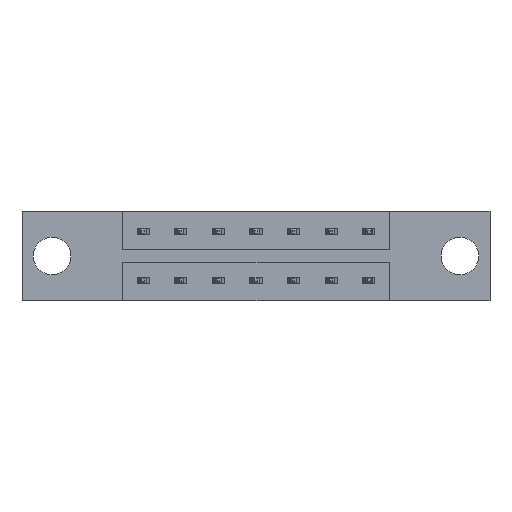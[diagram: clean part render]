
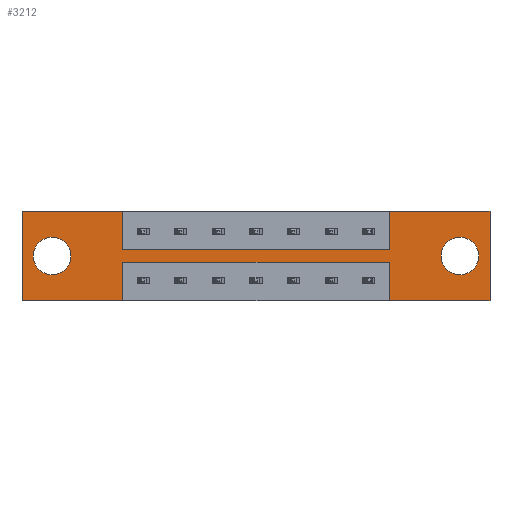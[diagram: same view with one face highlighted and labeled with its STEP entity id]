
A CAD part, front view. The second image highlights one B-rep face of the part: STEP entity #3212.
In plain terms, the highlighted planar face has unit normal (0, -1, 0).
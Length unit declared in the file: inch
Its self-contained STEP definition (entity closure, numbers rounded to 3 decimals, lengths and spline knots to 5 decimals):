
#24 = AXIS2_PLACEMENT_3D ( 'NONE', #7411, #3484, #8070 ) ;
#127 = VECTOR ( 'NONE', #6315, 39.37008 ) ;
#329 = CARTESIAN_POINT ( 'NONE',  ( 1.94, 0., 0. ) ) ;
#399 = VECTOR ( 'NONE', #4241, 39.37008 ) ;
#413 = VERTEX_POINT ( 'NONE', #4636 ) ;
#433 = DIRECTION ( 'NONE',  ( 0., 0., -1. ) ) ;
#529 = CARTESIAN_POINT ( 'NONE',  ( 1.5225, 0., -0.1585 ) ) ;
#573 = VECTOR ( 'NONE', #3287, 39.37008 ) ;
#631 = CIRCLE ( 'NONE', #5650, 0.078 ) ;
#705 = CARTESIAN_POINT ( 'NONE',  ( 1.815, 0., -0.107 ) ) ;
#706 = VERTEX_POINT ( 'NONE', #7564 ) ;
#843 = CARTESIAN_POINT ( 'NONE',  ( 0., 0., -0.37 ) ) ;
#888 = EDGE_LOOP ( 'NONE', ( #7225, #8269 ) ) ;
#948 = LINE ( 'NONE', #6165, #7922 ) ;
#1078 = DIRECTION ( 'NONE',  ( 0., 0., -1. ) ) ;
#1175 = DIRECTION ( 'NONE',  ( -1., 0., 0. ) ) ;
#1216 = DIRECTION ( 'NONE',  ( 0., 1., 0. ) ) ;
#1270 = VECTOR ( 'NONE', #6502, 39.37008 ) ;
#1649 = VERTEX_POINT ( 'NONE', #8091 ) ;
#1865 = DIRECTION ( 'NONE',  ( 0., 0., 1. ) ) ;
#1900 = CARTESIAN_POINT ( 'NONE',  ( 1.5225, 0., -0.1585 ) ) ;
#2024 = CARTESIAN_POINT ( 'NONE',  ( 0., 0., -0.37 ) ) ;
#2030 = EDGE_CURVE ( 'NONE', #2451, #5259, #2170, .T. ) ;
#2108 = EDGE_CURVE ( 'NONE', #413, #3306, #631, .T. ) ;
#2170 = CIRCLE ( 'NONE', #6915, 0.078 ) ;
#2182 = VERTEX_POINT ( 'NONE', #8765 ) ;
#2416 = EDGE_CURVE ( 'NONE', #5429, #7728, #8548, .T. ) ;
#2451 = VERTEX_POINT ( 'NONE', #6146 ) ;
#2578 = VERTEX_POINT ( 'NONE', #529 ) ;
#2615 = DIRECTION ( 'NONE',  ( 1., 0., 0. ) ) ;
#2626 = CARTESIAN_POINT ( 'NONE',  ( 1.5225, 0., 0. ) ) ;
#2696 = CARTESIAN_POINT ( 'NONE',  ( 0.4175, 0., -0.2115 ) ) ;
#2955 = LINE ( 'NONE', #7873, #573 ) ;
#3054 = EDGE_CURVE ( 'NONE', #1649, #3180, #4797, .T. ) ;
#3066 = CARTESIAN_POINT ( 'NONE',  ( 0.4175, 0., -0.1585 ) ) ;
#3070 = FACE_BOUND ( 'NONE', #8843, .T. ) ;
#3083 = EDGE_CURVE ( 'NONE', #5562, #1649, #6119, .T. ) ;
#3180 = VERTEX_POINT ( 'NONE', #6790 ) ;
#3212 = ADVANCED_FACE ( 'NONE', ( #8144, #3070, #3553 ), #8780, .T. ) ;
#3276 = VERTEX_POINT ( 'NONE', #7001 ) ;
#3287 = DIRECTION ( 'NONE',  ( 0., 0., -1. ) ) ;
#3306 = VERTEX_POINT ( 'NONE', #705 ) ;
#3331 = CARTESIAN_POINT ( 'NONE',  ( 0.125, 0., -0.107 ) ) ;
#3388 = EDGE_CURVE ( 'NONE', #2182, #706, #2955, .T. ) ;
#3434 = EDGE_CURVE ( 'NONE', #3180, #2578, #7637, .T. ) ;
#3484 = DIRECTION ( 'NONE',  ( 0., 1., 0. ) ) ;
#3522 = CIRCLE ( 'NONE', #24, 0.078 ) ;
#3553 = FACE_OUTER_BOUND ( 'NONE', #7498, .T. ) ;
#3596 = CARTESIAN_POINT ( 'NONE',  ( 0., 0., -0.37 ) ) ;
#3776 = EDGE_CURVE ( 'NONE', #3276, #6313, #8719, .T. ) ;
#3975 = LINE ( 'NONE', #2696, #5687 ) ;
#4093 = EDGE_CURVE ( 'NONE', #7728, #6301, #7932, .T. ) ;
#4158 = CARTESIAN_POINT ( 'NONE',  ( 1.815, 0., -0.185 ) ) ;
#4179 = CARTESIAN_POINT ( 'NONE',  ( 1.5225, 0., -0.2115 ) ) ;
#4241 = DIRECTION ( 'NONE',  ( -1., 0., 0. ) ) ;
#4394 = VECTOR ( 'NONE', #2615, 39.37008 ) ;
#4452 = ORIENTED_EDGE ( 'NONE', *, *, #6217, .T. ) ;
#4552 = LINE ( 'NONE', #5389, #7414 ) ;
#4625 = ORIENTED_EDGE ( 'NONE', *, *, #4093, .F. ) ;
#4636 = CARTESIAN_POINT ( 'NONE',  ( 1.815, 0., -0.263 ) ) ;
#4757 = ORIENTED_EDGE ( 'NONE', *, *, #2030, .T. ) ;
#4797 = LINE ( 'NONE', #3066, #8243 ) ;
#4800 = DIRECTION ( 'NONE',  ( 0., 0., -1. ) ) ;
#4918 = DIRECTION ( 'NONE',  ( 0., -1., 0. ) ) ;
#5007 = VECTOR ( 'NONE', #8396, 39.37008 ) ;
#5046 = ORIENTED_EDGE ( 'NONE', *, *, #3083, .F. ) ;
#5259 = VERTEX_POINT ( 'NONE', #3331 ) ;
#5311 = VECTOR ( 'NONE', #7405, 39.37008 ) ;
#5352 = EDGE_CURVE ( 'NONE', #7136, #5562, #4552, .T. ) ;
#5389 = CARTESIAN_POINT ( 'NONE',  ( 0., 0., 0. ) ) ;
#5429 = VERTEX_POINT ( 'NONE', #2626 ) ;
#5483 = LINE ( 'NONE', #1900, #7217 ) ;
#5510 = EDGE_CURVE ( 'NONE', #2578, #5429, #5483, .T. ) ;
#5562 = VERTEX_POINT ( 'NONE', #6705 ) ;
#5593 = EDGE_CURVE ( 'NONE', #6313, #2182, #3975, .T. ) ;
#5650 = AXIS2_PLACEMENT_3D ( 'NONE', #5690, #1216, #1078 ) ;
#5664 = CARTESIAN_POINT ( 'NONE',  ( 1.94, 0., 0. ) ) ;
#5687 = VECTOR ( 'NONE', #7394, 39.37008 ) ;
#5690 = CARTESIAN_POINT ( 'NONE',  ( 1.815, 0., -0.185 ) ) ;
#5768 = ORIENTED_EDGE ( 'NONE', *, *, #2416, .F. ) ;
#5982 = AXIS2_PLACEMENT_3D ( 'NONE', #3596, #4918, #433 ) ;
#6011 = CARTESIAN_POINT ( 'NONE',  ( 0.4175, 0., -0.1585 ) ) ;
#6119 = LINE ( 'NONE', #9014, #5007 ) ;
#6132 = CARTESIAN_POINT ( 'NONE',  ( 1.94, 0., -0.37 ) ) ;
#6146 = CARTESIAN_POINT ( 'NONE',  ( 0.125, 0., -0.263 ) ) ;
#6155 = EDGE_CURVE ( 'NONE', #3306, #413, #8709, .T. ) ;
#6165 = CARTESIAN_POINT ( 'NONE',  ( 0., 0., -0.37 ) ) ;
#6193 = LINE ( 'NONE', #2024, #399 ) ;
#6217 = EDGE_CURVE ( 'NONE', #5259, #2451, #3522, .T. ) ;
#6301 = VERTEX_POINT ( 'NONE', #6132 ) ;
#6313 = VERTEX_POINT ( 'NONE', #8095 ) ;
#6315 = DIRECTION ( 'NONE',  ( 0., 0., -1. ) ) ;
#6334 = EDGE_CURVE ( 'NONE', #706, #7136, #948, .T. ) ;
#6374 = EDGE_CURVE ( 'NONE', #6301, #3276, #6193, .T. ) ;
#6502 = DIRECTION ( 'NONE',  ( 1., 0., 0. ) ) ;
#6556 = CARTESIAN_POINT ( 'NONE',  ( 0., 0., 0. ) ) ;
#6611 = DIRECTION ( 'NONE',  ( 0., 1., 0. ) ) ;
#6619 = CARTESIAN_POINT ( 'NONE',  ( 0.125, 0., -0.185 ) ) ;
#6705 = CARTESIAN_POINT ( 'NONE',  ( 0., 0., 0. ) ) ;
#6790 = CARTESIAN_POINT ( 'NONE',  ( 0.4175, 0., -0.1585 ) ) ;
#6816 = DIRECTION ( 'NONE',  ( 0., 0., 1. ) ) ;
#6915 = AXIS2_PLACEMENT_3D ( 'NONE', #6619, #6611, #6816 ) ;
#7001 = CARTESIAN_POINT ( 'NONE',  ( 1.5225, 0., -0.37 ) ) ;
#7002 = ORIENTED_EDGE ( 'NONE', *, *, #6334, .F. ) ;
#7136 = VERTEX_POINT ( 'NONE', #843 ) ;
#7154 = ORIENTED_EDGE ( 'NONE', *, *, #3054, .F. ) ;
#7171 = ORIENTED_EDGE ( 'NONE', *, *, #5593, .F. ) ;
#7217 = VECTOR ( 'NONE', #8023, 39.37008 ) ;
#7225 = ORIENTED_EDGE ( 'NONE', *, *, #6155, .T. ) ;
#7327 = ORIENTED_EDGE ( 'NONE', *, *, #5510, .F. ) ;
#7394 = DIRECTION ( 'NONE',  ( -1., 0., 0. ) ) ;
#7405 = DIRECTION ( 'NONE',  ( 0., 0., 1. ) ) ;
#7411 = CARTESIAN_POINT ( 'NONE',  ( 0.125, 0., -0.185 ) ) ;
#7414 = VECTOR ( 'NONE', #1865, 39.37008 ) ;
#7498 = EDGE_LOOP ( 'NONE', ( #8449, #8585, #4625, #5768, #7327, #8587, #7154, #5046, #8338, #7002, #8535, #7171 ) ) ;
#7564 = CARTESIAN_POINT ( 'NONE',  ( 0.4175, 0., -0.37 ) ) ;
#7637 = LINE ( 'NONE', #6011, #4394 ) ;
#7705 = DIRECTION ( 'NONE',  ( 0., 0., -1. ) ) ;
#7728 = VERTEX_POINT ( 'NONE', #329 ) ;
#7873 = CARTESIAN_POINT ( 'NONE',  ( 0.4175, 0., -0.2115 ) ) ;
#7922 = VECTOR ( 'NONE', #1175, 39.37008 ) ;
#7932 = LINE ( 'NONE', #5664, #127 ) ;
#8023 = DIRECTION ( 'NONE',  ( 0., 0., 1. ) ) ;
#8070 = DIRECTION ( 'NONE',  ( 0., 0., 1. ) ) ;
#8091 = CARTESIAN_POINT ( 'NONE',  ( 0.4175, 0., 0. ) ) ;
#8095 = CARTESIAN_POINT ( 'NONE',  ( 1.5225, 0., -0.2115 ) ) ;
#8144 = FACE_BOUND ( 'NONE', #888, .T. ) ;
#8243 = VECTOR ( 'NONE', #7705, 39.37008 ) ;
#8269 = ORIENTED_EDGE ( 'NONE', *, *, #2108, .T. ) ;
#8338 = ORIENTED_EDGE ( 'NONE', *, *, #5352, .F. ) ;
#8396 = DIRECTION ( 'NONE',  ( 1., 0., 0. ) ) ;
#8449 = ORIENTED_EDGE ( 'NONE', *, *, #3776, .F. ) ;
#8535 = ORIENTED_EDGE ( 'NONE', *, *, #3388, .F. ) ;
#8548 = LINE ( 'NONE', #6556, #1270 ) ;
#8585 = ORIENTED_EDGE ( 'NONE', *, *, #6374, .F. ) ;
#8587 = ORIENTED_EDGE ( 'NONE', *, *, #3434, .F. ) ;
#8670 = DIRECTION ( 'NONE',  ( 0., 1., 0. ) ) ;
#8699 = AXIS2_PLACEMENT_3D ( 'NONE', #4158, #8670, #4800 ) ;
#8709 = CIRCLE ( 'NONE', #8699, 0.078 ) ;
#8719 = LINE ( 'NONE', #4179, #5311 ) ;
#8765 = CARTESIAN_POINT ( 'NONE',  ( 0.4175, 0., -0.2115 ) ) ;
#8780 = PLANE ( 'NONE',  #5982 ) ;
#8843 = EDGE_LOOP ( 'NONE', ( #4452, #4757 ) ) ;
#9014 = CARTESIAN_POINT ( 'NONE',  ( 0., 0., 0. ) ) ;
